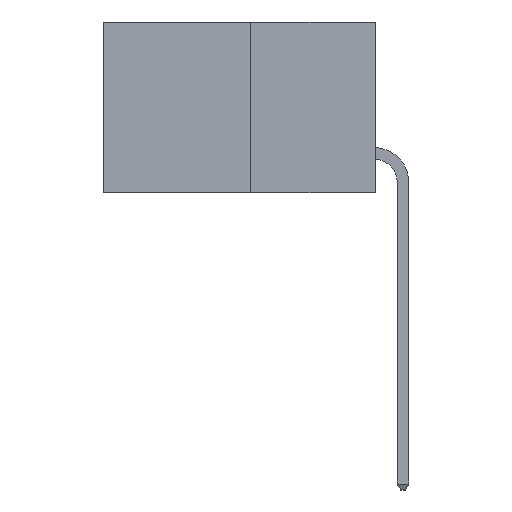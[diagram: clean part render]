
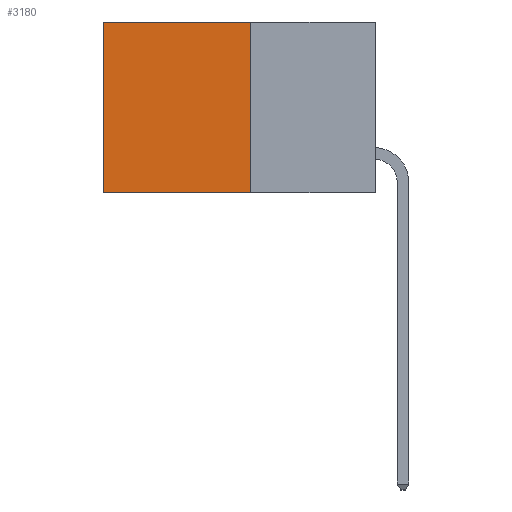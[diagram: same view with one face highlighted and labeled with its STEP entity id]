
A CAD part, left-side view. The second image highlights one B-rep face of the part: STEP entity #3180.
In plain terms, the highlighted planar face has unit normal (-1, 0, 0).
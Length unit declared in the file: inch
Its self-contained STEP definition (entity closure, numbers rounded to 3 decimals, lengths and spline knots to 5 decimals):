
#639 = CARTESIAN_POINT ( 'NONE',  ( 0.277, 0.27, -0.37 ) ) ;
#712 = FACE_OUTER_BOUND ( 'NONE', #19319, .T. ) ;
#938 = EDGE_CURVE ( 'NONE', #14991, #4816, #17495, .T. ) ;
#1093 = DIRECTION ( 'NONE',  ( 0., 0., -1. ) ) ;
#3180 = ADVANCED_FACE ( 'NONE', ( #712 ), #7662, .F. ) ;
#4214 = ORIENTED_EDGE ( 'NONE', *, *, #938, .F. ) ;
#4555 = VECTOR ( 'NONE', #14355, 39.37008 ) ;
#4797 = DIRECTION ( 'NONE',  ( 1., 0., 0. ) ) ;
#4816 = VERTEX_POINT ( 'NONE', #9997 ) ;
#6811 = EDGE_CURVE ( 'NONE', #7831, #14991, #18783, .T. ) ;
#7056 = CARTESIAN_POINT ( 'NONE',  ( 0.277, 0.59, -0.37 ) ) ;
#7662 = PLANE ( 'NONE',  #18971 ) ;
#7831 = VERTEX_POINT ( 'NONE', #12438 ) ;
#9260 = VECTOR ( 'NONE', #17617, 39.37008 ) ;
#9872 = CARTESIAN_POINT ( 'NONE',  ( 0.277, 0.27, -0.37 ) ) ;
#9997 = CARTESIAN_POINT ( 'NONE',  ( 0.277, 0.59, -0.37 ) ) ;
#10986 = EDGE_CURVE ( 'NONE', #7831, #12128, #12011, .T. ) ;
#11027 = VECTOR ( 'NONE', #11660, 39.37008 ) ;
#11405 = CARTESIAN_POINT ( 'NONE',  ( 0.277, 0.27, 0. ) ) ;
#11430 = LINE ( 'NONE', #7056, #14872 ) ;
#11576 = DIRECTION ( 'NONE',  ( 0., 0., -1. ) ) ;
#11660 = DIRECTION ( 'NONE',  ( 0., 0., -1. ) ) ;
#12011 = LINE ( 'NONE', #11405, #4555 ) ;
#12128 = VERTEX_POINT ( 'NONE', #18543 ) ;
#12438 = CARTESIAN_POINT ( 'NONE',  ( 0.277, 0.27, 0. ) ) ;
#13278 = CARTESIAN_POINT ( 'NONE',  ( 0.277, 0.27, -0.37 ) ) ;
#13813 = ORIENTED_EDGE ( 'NONE', *, *, #6811, .F. ) ;
#13991 = ORIENTED_EDGE ( 'NONE', *, *, #10986, .T. ) ;
#14355 = DIRECTION ( 'NONE',  ( 0., 1., 0. ) ) ;
#14872 = VECTOR ( 'NONE', #11576, 39.37008 ) ;
#14991 = VERTEX_POINT ( 'NONE', #9872 ) ;
#15326 = CARTESIAN_POINT ( 'NONE',  ( 0.277, 0.27, -0.37 ) ) ;
#15530 = ORIENTED_EDGE ( 'NONE', *, *, #18884, .T. ) ;
#17495 = LINE ( 'NONE', #13278, #9260 ) ;
#17617 = DIRECTION ( 'NONE',  ( 0., 1., 0. ) ) ;
#18543 = CARTESIAN_POINT ( 'NONE',  ( 0.277, 0.59, 0. ) ) ;
#18783 = LINE ( 'NONE', #15326, #11027 ) ;
#18884 = EDGE_CURVE ( 'NONE', #12128, #4816, #11430, .T. ) ;
#18971 = AXIS2_PLACEMENT_3D ( 'NONE', #639, #4797, #1093 ) ;
#19319 = EDGE_LOOP ( 'NONE', ( #15530, #4214, #13813, #13991 ) ) ;
